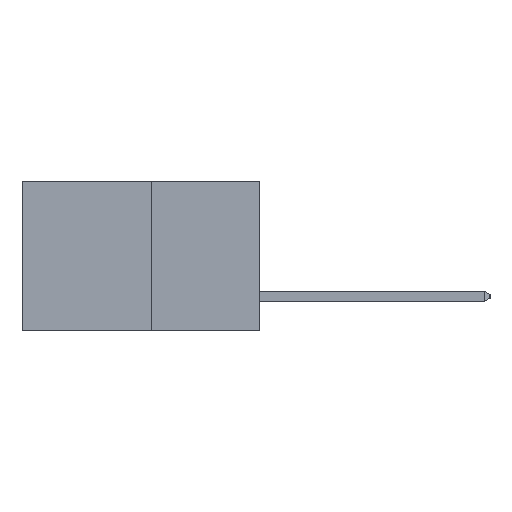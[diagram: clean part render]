
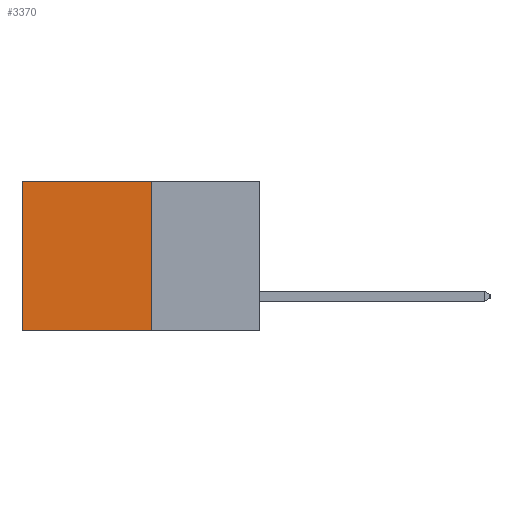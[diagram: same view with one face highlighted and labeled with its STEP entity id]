
A CAD part, left-side view. The second image highlights one B-rep face of the part: STEP entity #3370.
In plain terms, the highlighted planar face has unit normal (-1, 0, 0).
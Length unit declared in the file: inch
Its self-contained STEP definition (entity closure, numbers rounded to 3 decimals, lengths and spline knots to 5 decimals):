
#677 = VERTEX_POINT ( 'NONE', #1670 ) ;
#774 = DIRECTION ( 'NONE',  ( 0., 1., 0. ) ) ;
#836 = CARTESIAN_POINT ( 'NONE',  ( 0.277, 0.27, -0.37 ) ) ;
#1041 = EDGE_LOOP ( 'NONE', ( #2750, #2490, #3411, #2623 ) ) ;
#1122 = LINE ( 'NONE', #9272, #5278 ) ;
#1423 = CARTESIAN_POINT ( 'NONE',  ( 0.277, 0.27, 0. ) ) ;
#1670 = CARTESIAN_POINT ( 'NONE',  ( 0.277, 0.59, -0.37 ) ) ;
#1792 = FACE_OUTER_BOUND ( 'NONE', #1041, .T. ) ;
#2103 = DIRECTION ( 'NONE',  ( 0., 0., -1. ) ) ;
#2121 = EDGE_CURVE ( 'NONE', #3586, #677, #8229, .T. ) ;
#2447 = CARTESIAN_POINT ( 'NONE',  ( 0.277, 0.27, -0.37 ) ) ;
#2490 = ORIENTED_EDGE ( 'NONE', *, *, #7443, .F. ) ;
#2623 = ORIENTED_EDGE ( 'NONE', *, *, #2635, .T. ) ;
#2635 = EDGE_CURVE ( 'NONE', #6514, #3586, #1122, .T. ) ;
#2750 = ORIENTED_EDGE ( 'NONE', *, *, #2121, .T. ) ;
#2919 = LINE ( 'NONE', #836, #5276 ) ;
#3370 = ADVANCED_FACE ( 'NONE', ( #1792 ), #8354, .F. ) ;
#3411 = ORIENTED_EDGE ( 'NONE', *, *, #4042, .F. ) ;
#3586 = VERTEX_POINT ( 'NONE', #9466 ) ;
#4042 = EDGE_CURVE ( 'NONE', #6514, #7259, #9524, .T. ) ;
#5276 = VECTOR ( 'NONE', #774, 39.37008 ) ;
#5278 = VECTOR ( 'NONE', #8462, 39.37008 ) ;
#5571 = DIRECTION ( 'NONE',  ( 0., 0., -1. ) ) ;
#6514 = VERTEX_POINT ( 'NONE', #1423 ) ;
#6817 = CARTESIAN_POINT ( 'NONE',  ( 0.277, 0.27, -0.37 ) ) ;
#7048 = CARTESIAN_POINT ( 'NONE',  ( 0.277, 0.59, -0.37 ) ) ;
#7259 = VERTEX_POINT ( 'NONE', #2447 ) ;
#7443 = EDGE_CURVE ( 'NONE', #7259, #677, #2919, .T. ) ;
#7662 = VECTOR ( 'NONE', #2103, 39.37008 ) ;
#7762 = AXIS2_PLACEMENT_3D ( 'NONE', #7946, #8436, #8194 ) ;
#7946 = CARTESIAN_POINT ( 'NONE',  ( 0.277, 0.27, -0.37 ) ) ;
#8194 = DIRECTION ( 'NONE',  ( 0., 0., -1. ) ) ;
#8229 = LINE ( 'NONE', #7048, #9651 ) ;
#8354 = PLANE ( 'NONE',  #7762 ) ;
#8436 = DIRECTION ( 'NONE',  ( 1., 0., 0. ) ) ;
#8462 = DIRECTION ( 'NONE',  ( 0., 1., 0. ) ) ;
#9272 = CARTESIAN_POINT ( 'NONE',  ( 0.277, 0.27, 0. ) ) ;
#9466 = CARTESIAN_POINT ( 'NONE',  ( 0.277, 0.59, 0. ) ) ;
#9524 = LINE ( 'NONE', #6817, #7662 ) ;
#9651 = VECTOR ( 'NONE', #5571, 39.37008 ) ;
